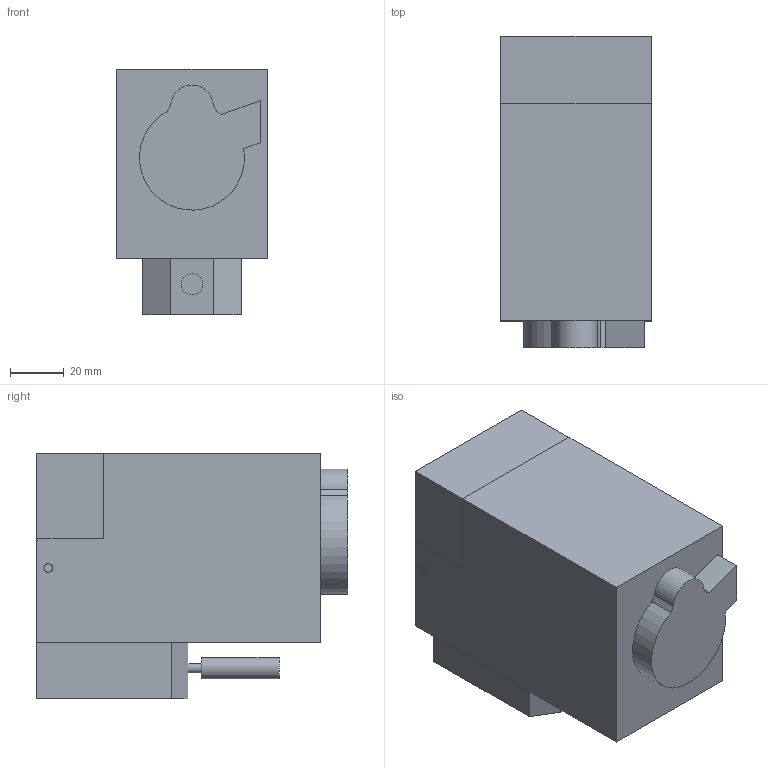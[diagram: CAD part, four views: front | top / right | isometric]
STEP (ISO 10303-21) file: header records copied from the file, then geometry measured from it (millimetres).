
FILE_DESCRIPTION(/* description */ (''),/* implementation_level */ '2;1');
FILE_NAME(/* name */ 'Tec9DevBlock.step',/* time_stamp */ '2025-05-27T11:15:51-07:00',/* author */ (''),/* organization */ (''),/* preprocessor_version */ 'ST-DEVELOPER v20.1',/* originating_system */ 'Autodesk Translation Framework v14.10.0.0',/* authorisation */ '');
FILE_SCHEMA (('AUTOMOTIVE_DESIGN { 1 0 10303 214 3 1 1 }'));
Length unit declared in the file: millimetre
Products named in the file (2): Tec9DragonMini; DragonDevBlock
Assembly tree (1 placements, depth 2):
  Tec9DragonMini
    DragonDevBlock
Bounding box: 56 x 116 x 91.57 mm (x, y, z)
Volume: 476690.9 mm3; surface area: 76422.6 mm2
Topology: 2 solids, 2 shells, 89 faces, 246 edges, 164 vertices
Faces by surface type: plane 69, cylinder 14, bspline 6
Full cylindrical faces by diameter (mm): 3.3 x4, 3.5 x1, 8 x1
Entity records: 3143 total; most frequent: CARTESIAN_POINT 801, ORIENTED_EDGE 492, DIRECTION 442, EDGE_CURVE 246, LINE 182, VECTOR 182, VERTEX_POINT 164, AXIS2_PLACEMENT_3D 130
